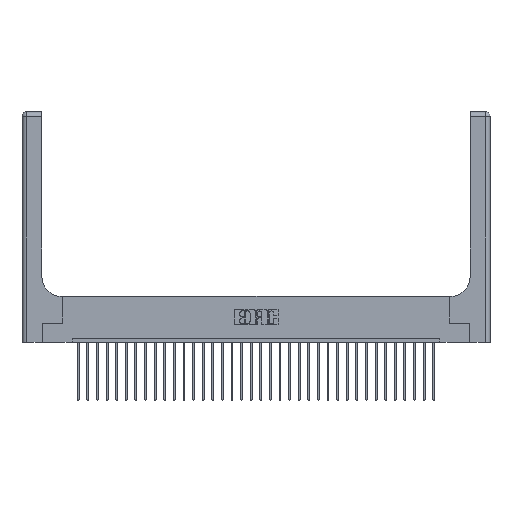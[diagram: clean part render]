
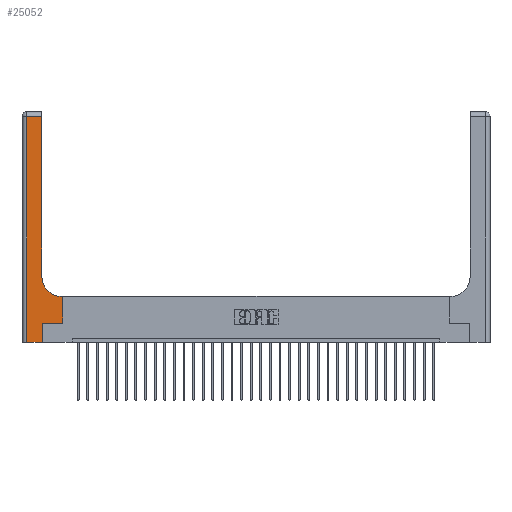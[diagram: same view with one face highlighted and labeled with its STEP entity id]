
A CAD part, top view. The second image highlights one B-rep face of the part: STEP entity #25052.
In plain terms, the highlighted planar face has unit normal (0, 0, 1).
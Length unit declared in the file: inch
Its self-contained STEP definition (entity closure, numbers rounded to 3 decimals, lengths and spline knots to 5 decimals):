
#42 = EDGE_CURVE ( 'NONE', #10902, #27619, #17006, .T. ) ;
#720 = VERTEX_POINT ( 'NONE', #19616 ) ;
#895 = CARTESIAN_POINT ( 'NONE',  ( 0.26, 3., 0.37 ) ) ;
#1609 = ORIENTED_EDGE ( 'NONE', *, *, #7903, .T. ) ;
#2089 = DIRECTION ( 'NONE',  ( 0., 0., -1. ) ) ;
#2821 = CARTESIAN_POINT ( 'NONE',  ( 0.265, 0., 0.37 ) ) ;
#3359 = DIRECTION ( 'NONE',  ( 0., 1., 0. ) ) ;
#3895 = VECTOR ( 'NONE', #11743, 39.37008 ) ;
#4045 = LINE ( 'NONE', #17735, #13102 ) ;
#5580 = DIRECTION ( 'NONE',  ( 1., 0., 0. ) ) ;
#5730 = ORIENTED_EDGE ( 'NONE', *, *, #16171, .T. ) ;
#6831 = DIRECTION ( 'NONE',  ( -1., 0., 0. ) ) ;
#7199 = VECTOR ( 'NONE', #9385, 39.37008 ) ;
#7335 = CARTESIAN_POINT ( 'NONE',  ( 0.06, 2.94, 0.37 ) ) ;
#7346 = VERTEX_POINT ( 'NONE', #16378 ) ;
#7864 = VERTEX_POINT ( 'NONE', #7335 ) ;
#7903 = EDGE_CURVE ( 'NONE', #22435, #720, #17204, .T. ) ;
#7931 = VECTOR ( 'NONE', #27746, 39.37008 ) ;
#8113 = CARTESIAN_POINT ( 'NONE',  ( 0.51, 0.6, 0.37 ) ) ;
#8330 = CARTESIAN_POINT ( 'NONE',  ( 0.06, 0., 0.37 ) ) ;
#8653 = CIRCLE ( 'NONE', #13461, 0.25 ) ;
#9102 = LINE ( 'NONE', #21096, #16795 ) ;
#9243 = ORIENTED_EDGE ( 'NONE', *, *, #12910, .T. ) ;
#9264 = LINE ( 'NONE', #895, #19492 ) ;
#9385 = DIRECTION ( 'NONE',  ( 1., 0., 0. ) ) ;
#9795 = EDGE_CURVE ( 'NONE', #7346, #22435, #16571, .T. ) ;
#10902 = VERTEX_POINT ( 'NONE', #8330 ) ;
#11311 = DIRECTION ( 'NONE',  ( 0., 0., -1. ) ) ;
#11394 = EDGE_CURVE ( 'NONE', #7864, #10902, #4045, .T. ) ;
#11743 = DIRECTION ( 'NONE',  ( 0., 1., 0. ) ) ;
#11760 = DIRECTION ( 'NONE',  ( 1., 0., 0. ) ) ;
#12359 = ORIENTED_EDGE ( 'NONE', *, *, #23573, .T. ) ;
#12910 = EDGE_CURVE ( 'NONE', #27619, #7346, #22842, .T. ) ;
#13102 = VECTOR ( 'NONE', #26738, 39.37008 ) ;
#13175 = VERTEX_POINT ( 'NONE', #8113 ) ;
#13461 = AXIS2_PLACEMENT_3D ( 'NONE', #23009, #11311, #11760 ) ;
#13993 = CARTESIAN_POINT ( 'NONE',  ( 0.528, 0.25, 0.37 ) ) ;
#14502 = ORIENTED_EDGE ( 'NONE', *, *, #11394, .T. ) ;
#14764 = ORIENTED_EDGE ( 'NONE', *, *, #23928, .T. ) ;
#16171 = EDGE_CURVE ( 'NONE', #720, #13175, #23394, .T. ) ;
#16258 = FACE_OUTER_BOUND ( 'NONE', #16683, .T. ) ;
#16378 = CARTESIAN_POINT ( 'NONE',  ( 0.265, 0.25, 0.37 ) ) ;
#16407 = CARTESIAN_POINT ( 'NONE',  ( 0., 3., 0.37 ) ) ;
#16571 = LINE ( 'NONE', #27827, #7199 ) ;
#16683 = EDGE_LOOP ( 'NONE', ( #24423, #12359, #14502, #18793, #9243, #21838, #1609, #5730, #14764 ) ) ;
#16795 = VECTOR ( 'NONE', #6831, 39.37008 ) ;
#16927 = CARTESIAN_POINT ( 'NONE',  ( 0.528, 0.25, 0.37 ) ) ;
#17006 = LINE ( 'NONE', #26166, #17825 ) ;
#17028 = DIRECTION ( 'NONE',  ( 0., 1., 0. ) ) ;
#17204 = LINE ( 'NONE', #16927, #22342 ) ;
#17735 = CARTESIAN_POINT ( 'NONE',  ( 0.06, 3., 0.37 ) ) ;
#17816 = EDGE_CURVE ( 'NONE', #28922, #22732, #9264, .T. ) ;
#17825 = VECTOR ( 'NONE', #5580, 39.37008 ) ;
#17831 = CARTESIAN_POINT ( 'NONE',  ( 0.265, 0., 0.37 ) ) ;
#18135 = CARTESIAN_POINT ( 'NONE',  ( 0.26, 0.85, 0.37 ) ) ;
#18503 = DIRECTION ( 'NONE',  ( -1., 0., 0. ) ) ;
#18580 = CARTESIAN_POINT ( 'NONE',  ( 0.26, 0.6, 0.37 ) ) ;
#18793 = ORIENTED_EDGE ( 'NONE', *, *, #42, .T. ) ;
#19492 = VECTOR ( 'NONE', #17028, 39.37008 ) ;
#19616 = CARTESIAN_POINT ( 'NONE',  ( 0.528, 0.6, 0.37 ) ) ;
#21096 = CARTESIAN_POINT ( 'NONE',  ( 0., 2.94, 0.37 ) ) ;
#21838 = ORIENTED_EDGE ( 'NONE', *, *, #9795, .T. ) ;
#22342 = VECTOR ( 'NONE', #3359, 39.37008 ) ;
#22435 = VERTEX_POINT ( 'NONE', #13993 ) ;
#22610 = AXIS2_PLACEMENT_3D ( 'NONE', #16407, #2089, #18503 ) ;
#22714 = PLANE ( 'NONE',  #22610 ) ;
#22732 = VERTEX_POINT ( 'NONE', #27309 ) ;
#22842 = LINE ( 'NONE', #2821, #3895 ) ;
#23009 = CARTESIAN_POINT ( 'NONE',  ( 0.51, 0.85, 0.37 ) ) ;
#23394 = LINE ( 'NONE', #18580, #7931 ) ;
#23573 = EDGE_CURVE ( 'NONE', #22732, #7864, #9102, .T. ) ;
#23928 = EDGE_CURVE ( 'NONE', #13175, #28922, #8653, .T. ) ;
#24423 = ORIENTED_EDGE ( 'NONE', *, *, #17816, .T. ) ;
#25052 = ADVANCED_FACE ( 'NONE', ( #16258 ), #22714, .F. ) ;
#26166 = CARTESIAN_POINT ( 'NONE',  ( 0., 0., 0.37 ) ) ;
#26738 = DIRECTION ( 'NONE',  ( 0., -1., 0. ) ) ;
#27309 = CARTESIAN_POINT ( 'NONE',  ( 0.26, 2.94, 0.37 ) ) ;
#27619 = VERTEX_POINT ( 'NONE', #17831 ) ;
#27746 = DIRECTION ( 'NONE',  ( -1., 0., 0. ) ) ;
#27827 = CARTESIAN_POINT ( 'NONE',  ( 0.265, 0.25, 0.37 ) ) ;
#28922 = VERTEX_POINT ( 'NONE', #18135 ) ;
